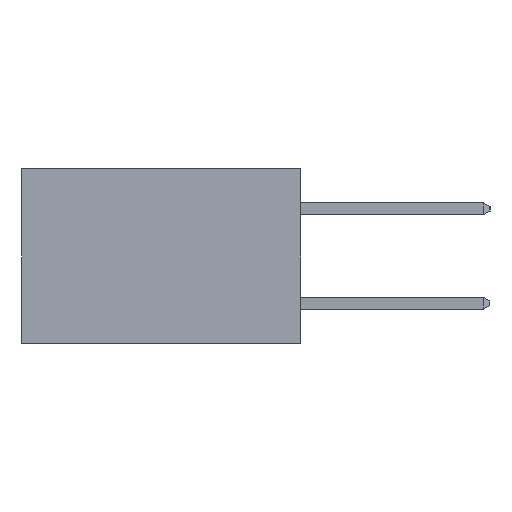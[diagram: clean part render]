
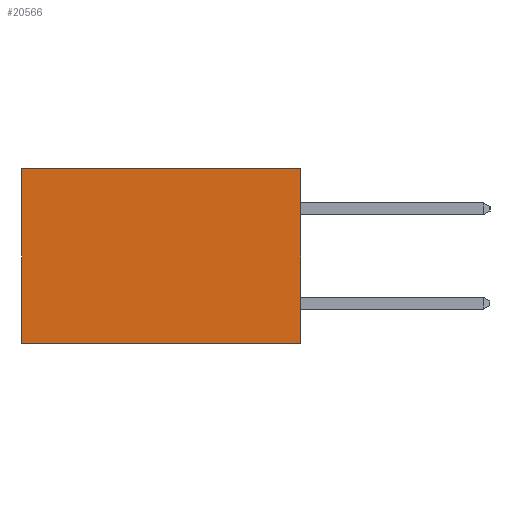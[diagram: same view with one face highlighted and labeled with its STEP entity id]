
A CAD part, left-side view. The second image highlights one B-rep face of the part: STEP entity #20566.
In plain terms, the highlighted planar face has unit normal (-1, 0, 0).
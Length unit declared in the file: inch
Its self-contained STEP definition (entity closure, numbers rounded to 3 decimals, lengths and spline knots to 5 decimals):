
#28 = VECTOR ( 'NONE', #13493, 39.37008 ) ;
#166 = LINE ( 'NONE', #3252, #7937 ) ;
#979 = EDGE_CURVE ( 'NONE', #19147, #1358, #10345, .T. ) ;
#1052 = EDGE_CURVE ( 'NONE', #3549, #19147, #8293, .T. ) ;
#1225 = ORIENTED_EDGE ( 'NONE', *, *, #3192, .T. ) ;
#1358 = VERTEX_POINT ( 'NONE', #18597 ) ;
#2089 = FACE_OUTER_BOUND ( 'NONE', #3591, .T. ) ;
#3192 = EDGE_CURVE ( 'NONE', #4079, #1358, #166, .T. ) ;
#3252 = CARTESIAN_POINT ( 'NONE',  ( 0.277, 0.59, -0.37 ) ) ;
#3413 = ORIENTED_EDGE ( 'NONE', *, *, #6200, .T. ) ;
#3549 = VERTEX_POINT ( 'NONE', #4590 ) ;
#3591 = EDGE_LOOP ( 'NONE', ( #1225, #9155, #8432, #3413 ) ) ;
#4079 = VERTEX_POINT ( 'NONE', #16961 ) ;
#4590 = CARTESIAN_POINT ( 'NONE',  ( 0.277, 0., 0. ) ) ;
#5246 = CARTESIAN_POINT ( 'NONE',  ( 0.277, 0., -0.37 ) ) ;
#5677 = CARTESIAN_POINT ( 'NONE',  ( 0.277, 0., -0.37 ) ) ;
#6200 = EDGE_CURVE ( 'NONE', #3549, #4079, #12079, .T. ) ;
#6240 = CARTESIAN_POINT ( 'NONE',  ( 0.277, 0., -0.37 ) ) ;
#6485 = CARTESIAN_POINT ( 'NONE',  ( 0.277, 0., 0. ) ) ;
#6515 = DIRECTION ( 'NONE',  ( 0., 1., 0. ) ) ;
#6838 = CARTESIAN_POINT ( 'NONE',  ( 0.277, 0., -0.37 ) ) ;
#7319 = VECTOR ( 'NONE', #6515, 39.37008 ) ;
#7937 = VECTOR ( 'NONE', #10278, 39.37008 ) ;
#8293 = LINE ( 'NONE', #5677, #28 ) ;
#8432 = ORIENTED_EDGE ( 'NONE', *, *, #1052, .F. ) ;
#9155 = ORIENTED_EDGE ( 'NONE', *, *, #979, .F. ) ;
#10072 = DIRECTION ( 'NONE',  ( 0., 0., -1. ) ) ;
#10278 = DIRECTION ( 'NONE',  ( 0., 0., -1. ) ) ;
#10345 = LINE ( 'NONE', #5246, #18372 ) ;
#12079 = LINE ( 'NONE', #6485, #7319 ) ;
#13493 = DIRECTION ( 'NONE',  ( 0., 0., -1. ) ) ;
#16961 = CARTESIAN_POINT ( 'NONE',  ( 0.277, 0.59, 0. ) ) ;
#18088 = PLANE ( 'NONE',  #20647 ) ;
#18372 = VECTOR ( 'NONE', #18760, 39.37008 ) ;
#18597 = CARTESIAN_POINT ( 'NONE',  ( 0.277, 0.59, -0.37 ) ) ;
#18760 = DIRECTION ( 'NONE',  ( 0., 1., 0. ) ) ;
#19147 = VERTEX_POINT ( 'NONE', #6240 ) ;
#19670 = DIRECTION ( 'NONE',  ( 1., 0., 0. ) ) ;
#20566 = ADVANCED_FACE ( 'NONE', ( #2089 ), #18088, .F. ) ;
#20647 = AXIS2_PLACEMENT_3D ( 'NONE', #6838, #19670, #10072 ) ;
